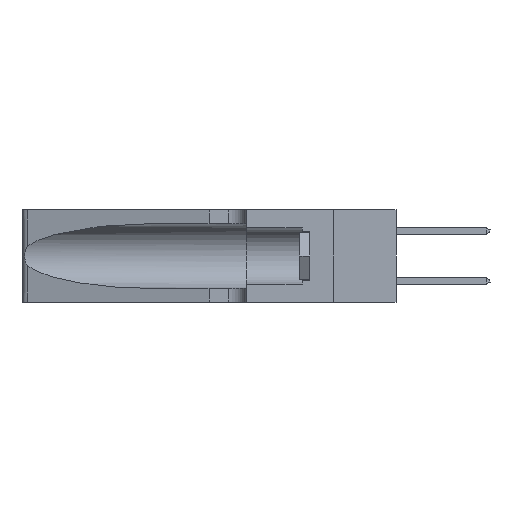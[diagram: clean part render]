
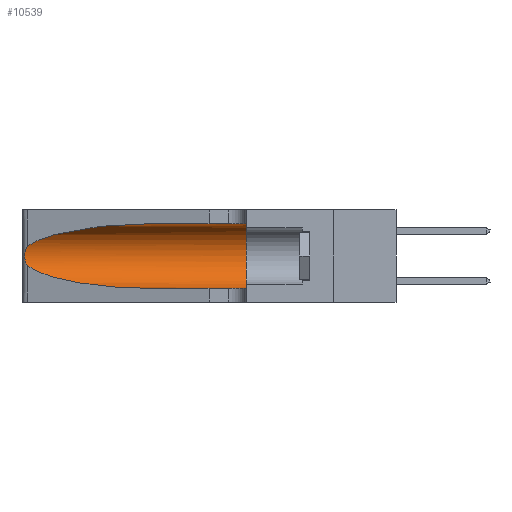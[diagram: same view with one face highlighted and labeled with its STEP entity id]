
A CAD part, left-side view. The second image highlights one B-rep face of the part: STEP entity #10539.
In plain terms, the highlighted cylindrical face has radius 3.308 mm (diameter 6.617 mm), a partial arc.
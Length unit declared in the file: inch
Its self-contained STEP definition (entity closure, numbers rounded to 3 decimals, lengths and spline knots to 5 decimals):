
#36 = CARTESIAN_POINT ( 'NONE',  ( 0.25487, 1.22718, 0.22369 ) ) ;
#383 = CARTESIAN_POINT ( 'NONE',  ( 0.26075, 1.23896, 0.19203 ) ) ;
#1739 = CARTESIAN_POINT ( 'NONE',  ( 0.18966, 0.96281, 0.05475 ) ) ;
#1901 = ORIENTED_EDGE ( 'NONE', *, *, #23824, .F. ) ;
#2356 = CARTESIAN_POINT ( 'NONE',  ( 0.26017, 1.23833, 0.17102 ) ) ;
#2396 = CARTESIAN_POINT ( 'NONE',  ( 0.1305, 0.72297, 0.05475 ) ) ;
#2652 = VERTEX_POINT ( 'NONE', #8265 ) ;
#2792 = CARTESIAN_POINT ( 'NONE',  ( 0.1305, 0.72297, 0.31525 ) ) ;
#3877 = DIRECTION ( 'NONE',  ( 0., -1., 0. ) ) ;
#4168 = EDGE_LOOP ( 'NONE', ( #11143, #16266, #8999, #14920, #9207, #1901 ) ) ;
#4290 = CARTESIAN_POINT ( 'NONE',  ( 0.25789, 1.23486, 0.15765 ) ) ;
#4790 = VERTEX_POINT ( 'NONE', #6243 ) ;
#5911 = CARTESIAN_POINT ( 'NONE',  ( 0.1305, 0.35, 0.185 ) ) ;
#6135 = CARTESIAN_POINT ( 'NONE',  ( 0.25487, 1.22718, 0.22369 ) ) ;
#6208 = CARTESIAN_POINT ( 'NONE',  ( 0.25555, 1.22993, 0.14849 ) ) ;
#6243 = CARTESIAN_POINT ( 'NONE',  ( 0.25487, 1.22718, 0.14631 ) ) ;
#6704 = VERTEX_POINT ( 'NONE', #2396 ) ;
#6896 = VECTOR ( 'NONE', #3877, 39.37008 ) ;
#7495 = LINE ( 'NONE', #18737, #6896 ) ;
#7577 = EDGE_CURVE ( 'NONE', #13536, #8710, #12410, .T. ) ;
#7825 = DIRECTION ( 'NONE',  ( 0., 0., 1. ) ) ;
#8045 =( BOUNDED_CURVE ( )  B_SPLINE_CURVE ( 3, ( #22065, #13077, #1739, #14890 ),
 .UNSPECIFIED., .F., .F. ) 
 B_SPLINE_CURVE_WITH_KNOTS ( ( 4, 4 ),
 ( 3.44316, 4.71239 ),
 .UNSPECIFIED. ) 
 CURVE ( )  GEOMETRIC_REPRESENTATION_ITEM ( )  RATIONAL_B_SPLINE_CURVE ( ( 1., 0.87, 0.87, 1. ) ) 
 REPRESENTATION_ITEM ( '' )  );
#8053 = CARTESIAN_POINT ( 'NONE',  ( 0.25555, 1.22994, 0.2215 ) ) ;
#8214 = CARTESIAN_POINT ( 'NONE',  ( 0.1305, 0.35, 0.05475 ) ) ;
#8265 = CARTESIAN_POINT ( 'NONE',  ( 0.1305, 0.35, 0.31525 ) ) ;
#8371 = FACE_OUTER_BOUND ( 'NONE', #4168, .T. ) ;
#8600 = EDGE_CURVE ( 'NONE', #4790, #6704, #8045, .T. ) ;
#8710 = VERTEX_POINT ( 'NONE', #36 ) ;
#8999 = ORIENTED_EDGE ( 'NONE', *, *, #8600, .T. ) ;
#9030 = DIRECTION ( 'NONE',  ( 0., 0., -1. ) ) ;
#9207 = ORIENTED_EDGE ( 'NONE', *, *, #18224, .F. ) ;
#9974 = CARTESIAN_POINT ( 'NONE',  ( 0.25787, 1.23484, 0.2124 ) ) ;
#10539 = ADVANCED_FACE ( 'NONE', ( #8371 ), #12766, .F. ) ;
#10642 = B_SPLINE_CURVE_WITH_KNOTS ( 'NONE', 3,
 ( #6135, #8053, #20832, #9974, #22639, #11836, #383, #13671, #2356, #15494, #4290, #17328, #6208, #19133 ),
 .UNSPECIFIED., .F., .F.,
 ( 4, 2, 2, 2, 2, 2, 4 ),
 ( 0., 0.00027, 0.00053, 0.00107, 0.0016, 0.00187, 0.00214 ),
 .UNSPECIFIED. ) ;
#11143 = ORIENTED_EDGE ( 'NONE', *, *, #7577, .T. ) ;
#11303 = VERTEX_POINT ( 'NONE', #8214 ) ;
#11472 = VECTOR ( 'NONE', #18543, 39.37008 ) ;
#11836 = CARTESIAN_POINT ( 'NONE',  ( 0.26018, 1.23835, 0.19895 ) ) ;
#12038 = LINE ( 'NONE', #20344, #11472 ) ;
#12253 = CARTESIAN_POINT ( 'NONE',  ( 0.18966, 0.96281, 0.31525 ) ) ;
#12410 =( BOUNDED_CURVE ( )  B_SPLINE_CURVE ( 3, ( #2792, #12253, #17645, #15907 ),
 .UNSPECIFIED., .F., .F. ) 
 B_SPLINE_CURVE_WITH_KNOTS ( ( 4, 4 ),
 ( 1.5708, 2.84003 ),
 .UNSPECIFIED. ) 
 CURVE ( )  GEOMETRIC_REPRESENTATION_ITEM ( )  RATIONAL_B_SPLINE_CURVE ( ( 1., 0.87, 0.87, 1. ) ) 
 REPRESENTATION_ITEM ( '' )  );
#12766 = CYLINDRICAL_SURFACE ( 'NONE', #21569, 0.13025 ) ;
#13077 = CARTESIAN_POINT ( 'NONE',  ( 0.2373, 1.15595, 0.08982 ) ) ;
#13536 = VERTEX_POINT ( 'NONE', #14833 ) ;
#13671 = CARTESIAN_POINT ( 'NONE',  ( 0.26075, 1.23896, 0.178 ) ) ;
#14833 = CARTESIAN_POINT ( 'NONE',  ( 0.1305, 0.72297, 0.31525 ) ) ;
#14890 = CARTESIAN_POINT ( 'NONE',  ( 0.1305, 0.72297, 0.05475 ) ) ;
#14920 = ORIENTED_EDGE ( 'NONE', *, *, #20464, .T. ) ;
#15008 = EDGE_CURVE ( 'NONE', #8710, #4790, #10642, .T. ) ;
#15494 = CARTESIAN_POINT ( 'NONE',  ( 0.25856, 1.23593, 0.16098 ) ) ;
#15907 = CARTESIAN_POINT ( 'NONE',  ( 0.25487, 1.22718, 0.22369 ) ) ;
#16266 = ORIENTED_EDGE ( 'NONE', *, *, #15008, .T. ) ;
#16332 = CARTESIAN_POINT ( 'NONE',  ( 0.1305, 1.61858, 0.185 ) ) ;
#16408 = DIRECTION ( 'NONE',  ( 0., -1., 0. ) ) ;
#17328 = CARTESIAN_POINT ( 'NONE',  ( 0.25639, 1.23186, 0.15144 ) ) ;
#17373 = AXIS2_PLACEMENT_3D ( 'NONE', #5911, #18837, #7825 ) ;
#17645 = CARTESIAN_POINT ( 'NONE',  ( 0.2373, 1.15595, 0.28018 ) ) ;
#18224 = EDGE_CURVE ( 'NONE', #2652, #11303, #22737, .T. ) ;
#18543 = DIRECTION ( 'NONE',  ( 0., -1., 0. ) ) ;
#18737 = CARTESIAN_POINT ( 'NONE',  ( 0.1305, 1.61858, 0.05475 ) ) ;
#18837 = DIRECTION ( 'NONE',  ( 0., 1., 0. ) ) ;
#19133 = CARTESIAN_POINT ( 'NONE',  ( 0.25487, 1.22718, 0.14631 ) ) ;
#20344 = CARTESIAN_POINT ( 'NONE',  ( 0.1305, 1.61858, 0.31525 ) ) ;
#20464 = EDGE_CURVE ( 'NONE', #6704, #11303, #7495, .T. ) ;
#20832 = CARTESIAN_POINT ( 'NONE',  ( 0.25639, 1.23184, 0.21858 ) ) ;
#21569 = AXIS2_PLACEMENT_3D ( 'NONE', #16332, #16408, #9030 ) ;
#22065 = CARTESIAN_POINT ( 'NONE',  ( 0.25487, 1.22718, 0.14631 ) ) ;
#22639 = CARTESIAN_POINT ( 'NONE',  ( 0.25854, 1.2359, 0.20912 ) ) ;
#22737 = CIRCLE ( 'NONE', #17373, 0.13025 ) ;
#23824 = EDGE_CURVE ( 'NONE', #13536, #2652, #12038, .T. ) ;
